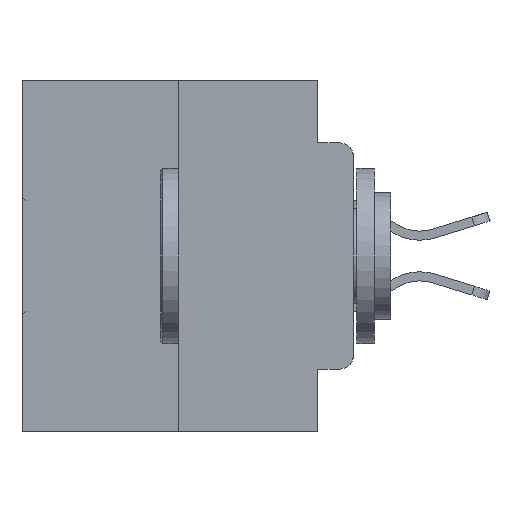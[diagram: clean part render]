
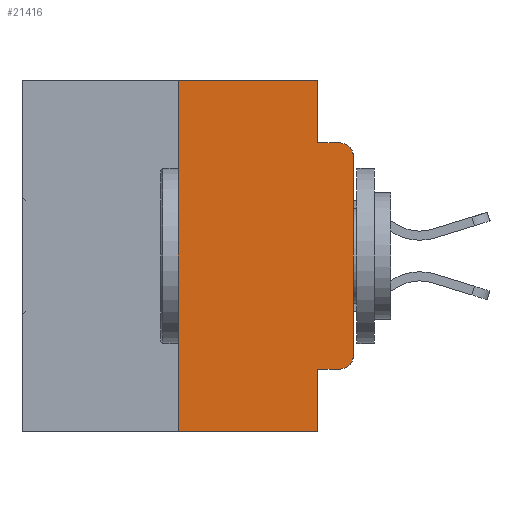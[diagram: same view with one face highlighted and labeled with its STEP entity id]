
A CAD part, left-side view. The second image highlights one B-rep face of the part: STEP entity #21416.
In plain terms, the highlighted planar face has unit normal (-1, 0, 0).
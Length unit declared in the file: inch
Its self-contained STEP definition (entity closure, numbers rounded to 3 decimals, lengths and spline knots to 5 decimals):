
#50 = VERTEX_POINT ( 'NONE', #23731 ) ;
#209 = CARTESIAN_POINT ( 'NONE',  ( 0., 0.473, 0. ) ) ;
#448 = VECTOR ( 'NONE', #24025, 39.37008 ) ;
#462 = VERTEX_POINT ( 'NONE', #11290 ) ;
#1219 = EDGE_CURVE ( 'NONE', #462, #26315, #10173, .T. ) ;
#1598 = DIRECTION ( 'NONE',  ( 0., -1., 0. ) ) ;
#1837 = ORIENTED_EDGE ( 'NONE', *, *, #2293, .T. ) ;
#1906 = DIRECTION ( 'NONE',  ( 0., 0., -1. ) ) ;
#2217 = AXIS2_PLACEMENT_3D ( 'NONE', #29893, #30218, #27371 ) ;
#2293 = EDGE_CURVE ( 'NONE', #6665, #21549, #29026, .T. ) ;
#3620 = ORIENTED_EDGE ( 'NONE', *, *, #1219, .F. ) ;
#3746 = VERTEX_POINT ( 'NONE', #14396 ) ;
#3793 = LINE ( 'NONE', #19132, #18523 ) ;
#4265 = CARTESIAN_POINT ( 'NONE',  ( 0., 0.051, 0. ) ) ;
#5379 = VERTEX_POINT ( 'NONE', #6114 ) ;
#6042 = CARTESIAN_POINT ( 'NONE',  ( 0., 0.051, -0.0885 ) ) ;
#6114 = CARTESIAN_POINT ( 'NONE',  ( 0., 0.051, -0.0885 ) ) ;
#6170 = ORIENTED_EDGE ( 'NONE', *, *, #21737, .F. ) ;
#6279 = VERTEX_POINT ( 'NONE', #14280 ) ;
#6557 = VECTOR ( 'NONE', #1906, 39.37008 ) ;
#6665 = VERTEX_POINT ( 'NONE', #32765 ) ;
#7209 = DIRECTION ( 'NONE',  ( 1., 0., 0. ) ) ;
#7299 = DIRECTION ( 'NONE',  ( 0., 0., 1. ) ) ;
#7998 = EDGE_CURVE ( 'NONE', #24279, #462, #14562, .T. ) ;
#10173 = LINE ( 'NONE', #209, #28195 ) ;
#11046 = ORIENTED_EDGE ( 'NONE', *, *, #17782, .T. ) ;
#11290 = CARTESIAN_POINT ( 'NONE',  ( 0., 0.25, 0. ) ) ;
#11736 = DIRECTION ( 'NONE',  ( 0., 0., -1. ) ) ;
#12745 = CARTESIAN_POINT ( 'NONE',  ( 0., 0.473, 0. ) ) ;
#12914 = DIRECTION ( 'NONE',  ( 0., 0., -1. ) ) ;
#13595 = CARTESIAN_POINT ( 'NONE',  ( 0., 0.051, 0. ) ) ;
#13771 = CARTESIAN_POINT ( 'NONE',  ( 0., 0.051, -0.4115 ) ) ;
#14280 = CARTESIAN_POINT ( 'NONE',  ( 0., 0., -0.3915 ) ) ;
#14396 = CARTESIAN_POINT ( 'NONE',  ( 0., 0.051, -0.5 ) ) ;
#14562 = LINE ( 'NONE', #28083, #26976 ) ;
#15097 = CARTESIAN_POINT ( 'NONE',  ( 0., 0.02, -0.4115 ) ) ;
#16140 = LINE ( 'NONE', #6042, #448 ) ;
#16457 = DIRECTION ( 'NONE',  ( 0., -1., 0. ) ) ;
#16849 = AXIS2_PLACEMENT_3D ( 'NONE', #12745, #7209, #28000 ) ;
#17782 = EDGE_CURVE ( 'NONE', #23961, #50, #17808, .T. ) ;
#17808 = CIRCLE ( 'NONE', #2217, 0.02 ) ;
#18523 = VECTOR ( 'NONE', #11736, 39.37008 ) ;
#19132 = CARTESIAN_POINT ( 'NONE',  ( 0., 0.051, 0. ) ) ;
#19548 = ORIENTED_EDGE ( 'NONE', *, *, #28851, .T. ) ;
#19754 = LINE ( 'NONE', #4265, #6557 ) ;
#20074 = LINE ( 'NONE', #30285, #29089 ) ;
#20169 = DIRECTION ( 'NONE',  ( -1., 0., 0. ) ) ;
#20208 = CARTESIAN_POINT ( 'NONE',  ( 0., 0.25, -0.5 ) ) ;
#20231 = DIRECTION ( 'NONE',  ( 0., 0., 1. ) ) ;
#20655 = CARTESIAN_POINT ( 'NONE',  ( 0., 0.02, -0.3915 ) ) ;
#20685 = ORIENTED_EDGE ( 'NONE', *, *, #26865, .T. ) ;
#21416 = ADVANCED_FACE ( 'NONE', ( #33026 ), #26590, .F. ) ;
#21549 = VERTEX_POINT ( 'NONE', #15097 ) ;
#21737 = EDGE_CURVE ( 'NONE', #6665, #3746, #3793, .T. ) ;
#22428 = EDGE_LOOP ( 'NONE', ( #25253, #11046, #31759, #28918, #3620, #29573, #20685, #6170, #1837, #19548 ) ) ;
#22496 = AXIS2_PLACEMENT_3D ( 'NONE', #20655, #20169, #12914 ) ;
#23545 = CIRCLE ( 'NONE', #22496, 0.02 ) ;
#23731 = CARTESIAN_POINT ( 'NONE',  ( 0., 0.02, -0.0885 ) ) ;
#23961 = VERTEX_POINT ( 'NONE', #31440 ) ;
#24025 = DIRECTION ( 'NONE',  ( 0., -1., 0. ) ) ;
#24077 = VECTOR ( 'NONE', #1598, 39.37008 ) ;
#24279 = VERTEX_POINT ( 'NONE', #20208 ) ;
#25253 = ORIENTED_EDGE ( 'NONE', *, *, #31901, .T. ) ;
#26315 = VERTEX_POINT ( 'NONE', #13595 ) ;
#26590 = PLANE ( 'NONE',  #16849 ) ;
#26796 = LINE ( 'NONE', #31819, #24077 ) ;
#26865 = EDGE_CURVE ( 'NONE', #24279, #3746, #26796, .T. ) ;
#26976 = VECTOR ( 'NONE', #20231, 39.37008 ) ;
#27371 = DIRECTION ( 'NONE',  ( 0., 0., -1. ) ) ;
#28000 = DIRECTION ( 'NONE',  ( 0., 0., -1. ) ) ;
#28083 = CARTESIAN_POINT ( 'NONE',  ( 0., 0.25, 0. ) ) ;
#28195 = VECTOR ( 'NONE', #28278, 39.37008 ) ;
#28278 = DIRECTION ( 'NONE',  ( 0., -1., 0. ) ) ;
#28653 = EDGE_CURVE ( 'NONE', #5379, #50, #16140, .T. ) ;
#28851 = EDGE_CURVE ( 'NONE', #21549, #6279, #23545, .T. ) ;
#28918 = ORIENTED_EDGE ( 'NONE', *, *, #31742, .F. ) ;
#29021 = VECTOR ( 'NONE', #16457, 39.37008 ) ;
#29026 = LINE ( 'NONE', #13771, #29021 ) ;
#29089 = VECTOR ( 'NONE', #7299, 39.37008 ) ;
#29573 = ORIENTED_EDGE ( 'NONE', *, *, #7998, .F. ) ;
#29893 = CARTESIAN_POINT ( 'NONE',  ( 0., 0.02, -0.1085 ) ) ;
#30218 = DIRECTION ( 'NONE',  ( -1., 0., 0. ) ) ;
#30285 = CARTESIAN_POINT ( 'NONE',  ( 0., 0., 0. ) ) ;
#31440 = CARTESIAN_POINT ( 'NONE',  ( 0., 0., -0.1085 ) ) ;
#31742 = EDGE_CURVE ( 'NONE', #26315, #5379, #19754, .T. ) ;
#31759 = ORIENTED_EDGE ( 'NONE', *, *, #28653, .F. ) ;
#31819 = CARTESIAN_POINT ( 'NONE',  ( 0., 0.473, -0.5 ) ) ;
#31901 = EDGE_CURVE ( 'NONE', #6279, #23961, #20074, .T. ) ;
#32765 = CARTESIAN_POINT ( 'NONE',  ( 0., 0.051, -0.4115 ) ) ;
#33026 = FACE_OUTER_BOUND ( 'NONE', #22428, .T. ) ;
